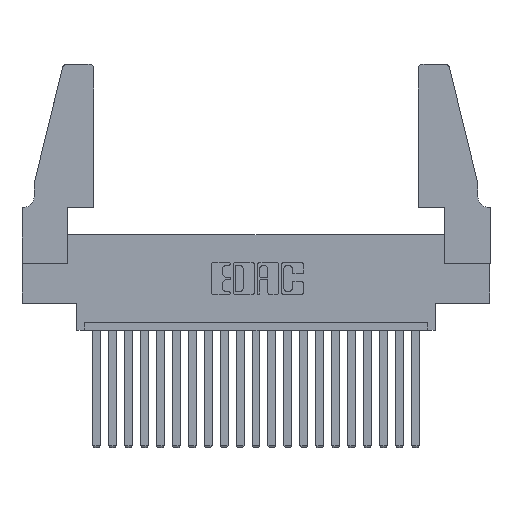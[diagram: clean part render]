
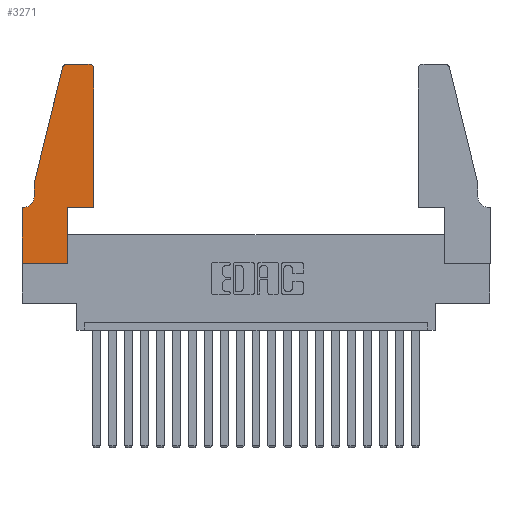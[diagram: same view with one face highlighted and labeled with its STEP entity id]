
A CAD part, top view. The second image highlights one B-rep face of the part: STEP entity #3271.
In plain terms, the highlighted planar face has unit normal (0, 0, 1).
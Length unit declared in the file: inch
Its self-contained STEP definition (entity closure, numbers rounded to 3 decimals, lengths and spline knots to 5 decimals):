
#130 = EDGE_CURVE ( 'NONE', #8807, #4834, #17797, .T. ) ;
#412 = VECTOR ( 'NONE', #7121, 39.37008 ) ;
#493 = VECTOR ( 'NONE', #10027, 39.37008 ) ;
#740 = VECTOR ( 'NONE', #1116, 39.37008 ) ;
#1015 = LINE ( 'NONE', #17477, #7546 ) ;
#1040 = LINE ( 'NONE', #12088, #8822 ) ;
#1067 = AXIS2_PLACEMENT_3D ( 'NONE', #19668, #6814, #19535 ) ;
#1116 = DIRECTION ( 'NONE',  ( -1., 0., 0. ) ) ;
#1446 = ORIENTED_EDGE ( 'NONE', *, *, #8927, .T. ) ;
#1563 = EDGE_CURVE ( 'NONE', #18425, #9394, #17006, .T. ) ;
#2001 = CIRCLE ( 'NONE', #20165, 0.03 ) ;
#2036 = ORIENTED_EDGE ( 'NONE', *, *, #16988, .T. ) ;
#3130 = LINE ( 'NONE', #11769, #493 ) ;
#3271 = ADVANCED_FACE ( 'NONE', ( #3407 ), #7014, .T. ) ;
#3407 = FACE_OUTER_BOUND ( 'NONE', #8843, .T. ) ;
#3626 = EDGE_CURVE ( 'NONE', #9394, #13064, #15673, .T. ) ;
#3656 = ORIENTED_EDGE ( 'NONE', *, *, #7088, .T. ) ;
#3988 = CARTESIAN_POINT ( 'NONE',  ( 0.2865, 0., 0.37 ) ) ;
#4518 = VECTOR ( 'NONE', #12364, 39.37008 ) ;
#4834 = VERTEX_POINT ( 'NONE', #13732 ) ;
#5122 = EDGE_CURVE ( 'NONE', #16812, #9282, #10345, .T. ) ;
#5673 = CARTESIAN_POINT ( 'NONE',  ( 0.4205, 1.22, 0.37 ) ) ;
#5817 = DIRECTION ( 'NONE',  ( 1., 0., 0. ) ) ;
#5933 = ORIENTED_EDGE ( 'NONE', *, *, #3626, .T. ) ;
#6166 = EDGE_CURVE ( 'NONE', #11779, #18425, #1040, .T. ) ;
#6258 = LINE ( 'NONE', #10274, #4518 ) ;
#6316 = EDGE_CURVE ( 'NONE', #20731, #15879, #1015, .T. ) ;
#6814 = DIRECTION ( 'NONE',  ( 0., 0., 1. ) ) ;
#6968 = VECTOR ( 'NONE', #17463, 39.37008 ) ;
#7014 = PLANE ( 'NONE',  #1067 ) ;
#7088 = EDGE_CURVE ( 'NONE', #9282, #20731, #6258, .T. ) ;
#7121 = DIRECTION ( 'NONE',  ( 0., -1., 0. ) ) ;
#7152 = EDGE_CURVE ( 'NONE', #4834, #11779, #2001, .T. ) ;
#7154 = CARTESIAN_POINT ( 'NONE',  ( 0.0055, 0.35, 0.37 ) ) ;
#7502 = ORIENTED_EDGE ( 'NONE', *, *, #6316, .T. ) ;
#7546 = VECTOR ( 'NONE', #7892, 39.37008 ) ;
#7619 = CARTESIAN_POINT ( 'NONE',  ( 0.4505, 0.35, 0.37 ) ) ;
#7781 = ORIENTED_EDGE ( 'NONE', *, *, #18255, .T. ) ;
#7881 = CARTESIAN_POINT ( 'NONE',  ( 0.4505, 1.22, 0.37 ) ) ;
#7892 = DIRECTION ( 'NONE',  ( 1., 0., 0. ) ) ;
#7893 = CARTESIAN_POINT ( 'NONE',  ( 0.2865, 0.35, 0.37 ) ) ;
#8047 = LINE ( 'NONE', #20167, #740 ) ;
#8517 = DIRECTION ( 'NONE',  ( -1., 0., 0. ) ) ;
#8595 = DIRECTION ( 'NONE',  ( 0., 0., -1. ) ) ;
#8807 = VERTEX_POINT ( 'NONE', #9320 ) ;
#8822 = VECTOR ( 'NONE', #18528, 39.37008 ) ;
#8843 = EDGE_LOOP ( 'NONE', ( #19353, #15519, #10507, #11014, #5933, #18460, #1446, #18041, #3656, #7502, #2036, #7781 ) ) ;
#8927 = EDGE_CURVE ( 'NONE', #14128, #16812, #10448, .T. ) ;
#9155 = CARTESIAN_POINT ( 'NONE',  ( 0.2605, 1.25, 0.37 ) ) ;
#9282 = VERTEX_POINT ( 'NONE', #3988 ) ;
#9320 = CARTESIAN_POINT ( 'NONE',  ( 0.4205, 1.25, 0.37 ) ) ;
#9394 = VERTEX_POINT ( 'NONE', #13212 ) ;
#9560 = CARTESIAN_POINT ( 'NONE',  ( 0.0755, 0.5, 0.37 ) ) ;
#10027 = DIRECTION ( 'NONE',  ( 0., 1., 0. ) ) ;
#10028 = VECTOR ( 'NONE', #12439, 39.37008 ) ;
#10265 = CARTESIAN_POINT ( 'NONE',  ( 0.0055, 0.42, 0.37 ) ) ;
#10274 = CARTESIAN_POINT ( 'NONE',  ( 0.2865, 0.35, 0.37 ) ) ;
#10345 = LINE ( 'NONE', #15930, #11855 ) ;
#10448 = LINE ( 'NONE', #10558, #412 ) ;
#10507 = ORIENTED_EDGE ( 'NONE', *, *, #6166, .T. ) ;
#10558 = CARTESIAN_POINT ( 'NONE',  ( 0., 0., 0.37 ) ) ;
#11014 = ORIENTED_EDGE ( 'NONE', *, *, #1563, .T. ) ;
#11214 = AXIS2_PLACEMENT_3D ( 'NONE', #5673, #15584, #5817 ) ;
#11713 = AXIS2_PLACEMENT_3D ( 'NONE', #10265, #8595, #8517 ) ;
#11748 = CARTESIAN_POINT ( 'NONE',  ( 0., 0.35, 0.37 ) ) ;
#11769 = CARTESIAN_POINT ( 'NONE',  ( 0.4505, 0.35, 0.37 ) ) ;
#11779 = VERTEX_POINT ( 'NONE', #16880 ) ;
#11855 = VECTOR ( 'NONE', #20589, 39.37008 ) ;
#12088 = CARTESIAN_POINT ( 'NONE',  ( 0.0755, 0.5, 0.37 ) ) ;
#12364 = DIRECTION ( 'NONE',  ( 0., 1., 0. ) ) ;
#12439 = DIRECTION ( 'NONE',  ( -1., 0., 0. ) ) ;
#12697 = CARTESIAN_POINT ( 'NONE',  ( 0.0755, 0.5, 0.37 ) ) ;
#13064 = VERTEX_POINT ( 'NONE', #7154 ) ;
#13179 = EDGE_CURVE ( 'NONE', #13064, #14128, #8047, .T. ) ;
#13212 = CARTESIAN_POINT ( 'NONE',  ( 0.0755, 0.42, 0.37 ) ) ;
#13407 = CIRCLE ( 'NONE', #11214, 0.03 ) ;
#13732 = CARTESIAN_POINT ( 'NONE',  ( 0.284, 1.25, 0.37 ) ) ;
#13931 = DIRECTION ( 'NONE',  ( 0., 0., 1. ) ) ;
#14128 = VERTEX_POINT ( 'NONE', #11748 ) ;
#15405 = DIRECTION ( 'NONE',  ( 1., 0., 0. ) ) ;
#15519 = ORIENTED_EDGE ( 'NONE', *, *, #7152, .T. ) ;
#15584 = DIRECTION ( 'NONE',  ( 0., 0., 1. ) ) ;
#15673 = CIRCLE ( 'NONE', #11713, 0.07 ) ;
#15879 = VERTEX_POINT ( 'NONE', #7619 ) ;
#15930 = CARTESIAN_POINT ( 'NONE',  ( 0., 0., 0.37 ) ) ;
#16427 = VERTEX_POINT ( 'NONE', #7881 ) ;
#16812 = VERTEX_POINT ( 'NONE', #18747 ) ;
#16880 = CARTESIAN_POINT ( 'NONE',  ( 0.25487, 1.22718, 0.37 ) ) ;
#16988 = EDGE_CURVE ( 'NONE', #15879, #16427, #3130, .T. ) ;
#17006 = LINE ( 'NONE', #12697, #6968 ) ;
#17463 = DIRECTION ( 'NONE',  ( 0., -1., 0. ) ) ;
#17477 = CARTESIAN_POINT ( 'NONE',  ( 0.4505, 0.35, 0.37 ) ) ;
#17797 = LINE ( 'NONE', #9155, #10028 ) ;
#18041 = ORIENTED_EDGE ( 'NONE', *, *, #5122, .T. ) ;
#18255 = EDGE_CURVE ( 'NONE', #16427, #8807, #13407, .T. ) ;
#18425 = VERTEX_POINT ( 'NONE', #9560 ) ;
#18460 = ORIENTED_EDGE ( 'NONE', *, *, #13179, .T. ) ;
#18528 = DIRECTION ( 'NONE',  ( -0.239, -0.971, 0. ) ) ;
#18747 = CARTESIAN_POINT ( 'NONE',  ( 0., 0., 0.37 ) ) ;
#19353 = ORIENTED_EDGE ( 'NONE', *, *, #130, .T. ) ;
#19535 = DIRECTION ( 'NONE',  ( 1., 0., 0. ) ) ;
#19668 = CARTESIAN_POINT ( 'NONE',  ( 0., 0.35, 0.37 ) ) ;
#20146 = CARTESIAN_POINT ( 'NONE',  ( 0.284, 1.22, 0.37 ) ) ;
#20165 = AXIS2_PLACEMENT_3D ( 'NONE', #20146, #13931, #15405 ) ;
#20167 = CARTESIAN_POINT ( 'NONE',  ( 0.0755, 0.35, 0.37 ) ) ;
#20589 = DIRECTION ( 'NONE',  ( 1., 0., 0. ) ) ;
#20731 = VERTEX_POINT ( 'NONE', #7893 ) ;
